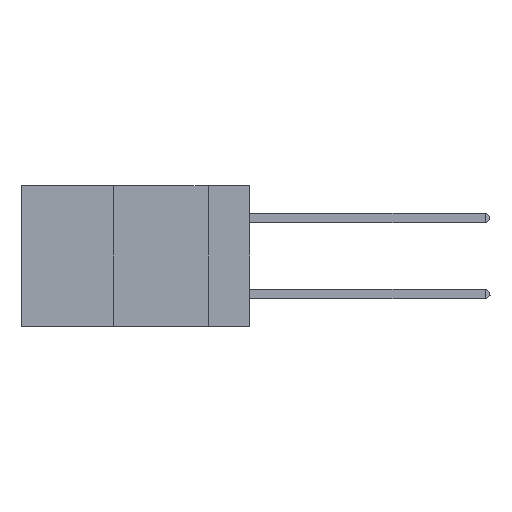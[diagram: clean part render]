
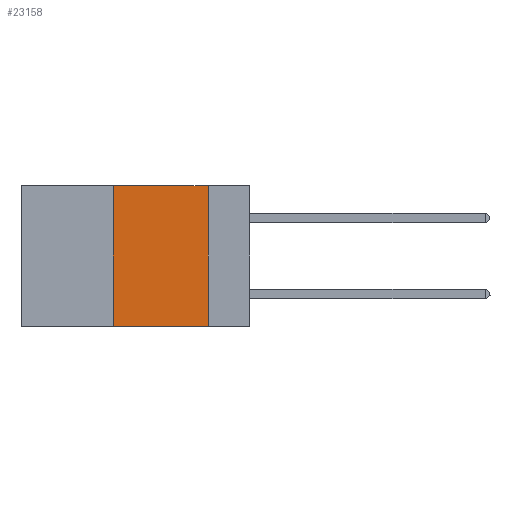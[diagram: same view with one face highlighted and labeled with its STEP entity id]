
A CAD part, left-side view. The second image highlights one B-rep face of the part: STEP entity #23158.
In plain terms, the highlighted planar face has unit normal (-1, 0, 0).
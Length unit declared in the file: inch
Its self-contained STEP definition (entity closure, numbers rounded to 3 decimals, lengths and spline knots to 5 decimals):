
#1017 = ORIENTED_EDGE ( 'NONE', *, *, #33917, .F. ) ;
#5155 = CARTESIAN_POINT ( 'NONE',  ( 0., 0.36, -0.37 ) ) ;
#5219 = LINE ( 'NONE', #33230, #35689 ) ;
#6252 = VECTOR ( 'NONE', #34281, 39.37008 ) ;
#12514 = ORIENTED_EDGE ( 'NONE', *, *, #15902, .F. ) ;
#14574 = CARTESIAN_POINT ( 'NONE',  ( 0., 0.36, 0. ) ) ;
#15268 = FACE_OUTER_BOUND ( 'NONE', #38029, .T. ) ;
#15902 = EDGE_CURVE ( 'NONE', #21996, #18635, #39507, .T. ) ;
#18635 = VERTEX_POINT ( 'NONE', #39110 ) ;
#19924 = VERTEX_POINT ( 'NONE', #30371 ) ;
#20557 = DIRECTION ( 'NONE',  ( 0., 0., 1. ) ) ;
#21996 = VERTEX_POINT ( 'NONE', #14574 ) ;
#22194 = DIRECTION ( 'NONE',  ( 0., 0., -1. ) ) ;
#22862 = CARTESIAN_POINT ( 'NONE',  ( 0., 0.6, 0. ) ) ;
#23158 = ADVANCED_FACE ( 'NONE', ( #15268 ), #39294, .F. ) ;
#25442 = VERTEX_POINT ( 'NONE', #5155 ) ;
#26990 = DIRECTION ( 'NONE',  ( 0., -1., 0. ) ) ;
#28929 = CARTESIAN_POINT ( 'NONE',  ( 0., 0.11, 0. ) ) ;
#29455 = DIRECTION ( 'NONE',  ( 1., 0., 0. ) ) ;
#30225 = AXIS2_PLACEMENT_3D ( 'NONE', #22862, #29455, #39437 ) ;
#30298 = CARTESIAN_POINT ( 'NONE',  ( 0., 0.6, 0. ) ) ;
#30312 = ORIENTED_EDGE ( 'NONE', *, *, #40636, .F. ) ;
#30371 = CARTESIAN_POINT ( 'NONE',  ( 0., 0.11, -0.37 ) ) ;
#31582 = VECTOR ( 'NONE', #22194, 39.37008 ) ;
#32116 = EDGE_CURVE ( 'NONE', #25442, #19924, #34164, .T. ) ;
#33230 = CARTESIAN_POINT ( 'NONE',  ( 0., 0.36, 0. ) ) ;
#33917 = EDGE_CURVE ( 'NONE', #18635, #19924, #39341, .T. ) ;
#34164 = LINE ( 'NONE', #37323, #6252 ) ;
#34281 = DIRECTION ( 'NONE',  ( 0., -1., 0. ) ) ;
#35689 = VECTOR ( 'NONE', #20557, 39.37008 ) ;
#36386 = VECTOR ( 'NONE', #26990, 39.37008 ) ;
#37323 = CARTESIAN_POINT ( 'NONE',  ( 0., 0.6, -0.37 ) ) ;
#38029 = EDGE_LOOP ( 'NONE', ( #1017, #12514, #30312, #39489 ) ) ;
#39110 = CARTESIAN_POINT ( 'NONE',  ( 0., 0.11, 0. ) ) ;
#39294 = PLANE ( 'NONE',  #30225 ) ;
#39341 = LINE ( 'NONE', #28929, #31582 ) ;
#39437 = DIRECTION ( 'NONE',  ( 0., 0., -1. ) ) ;
#39489 = ORIENTED_EDGE ( 'NONE', *, *, #32116, .T. ) ;
#39507 = LINE ( 'NONE', #30298, #36386 ) ;
#40636 = EDGE_CURVE ( 'NONE', #25442, #21996, #5219, .T. ) ;
